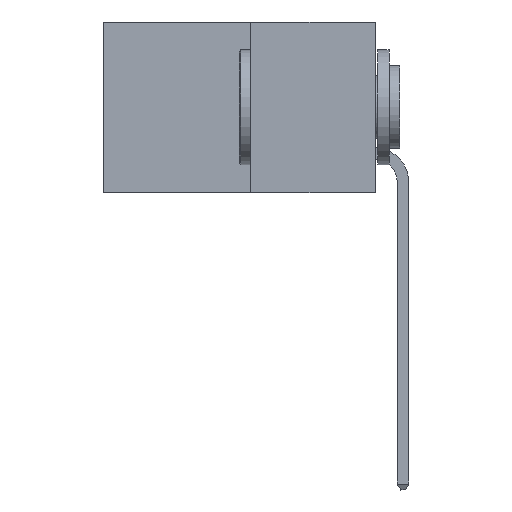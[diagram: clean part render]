
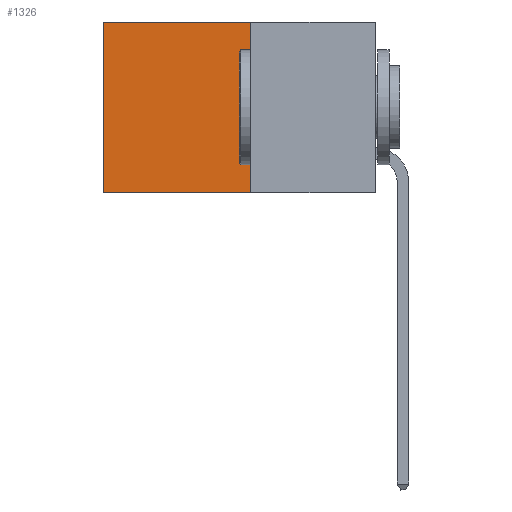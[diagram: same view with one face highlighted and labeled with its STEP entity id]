
A CAD part, left-side view. The second image highlights one B-rep face of the part: STEP entity #1326.
In plain terms, the highlighted planar face has unit normal (-1, 0, 0).
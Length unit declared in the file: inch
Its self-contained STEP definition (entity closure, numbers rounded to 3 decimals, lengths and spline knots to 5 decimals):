
#985 = AXIS2_PLACEMENT_3D ( 'NONE', #12984, #8369, #6080 ) ;
#992 = CARTESIAN_POINT ( 'NONE',  ( 0.277, 0.59, 0. ) ) ;
#1101 = VERTEX_POINT ( 'NONE', #992 ) ;
#1326 = ADVANCED_FACE ( 'NONE', ( #7805 ), #9243, .F. ) ;
#1592 = DIRECTION ( 'NONE',  ( 0., 1., 0. ) ) ;
#2831 = LINE ( 'NONE', #6170, #10589 ) ;
#2995 = VECTOR ( 'NONE', #11701, 39.37008 ) ;
#3074 = EDGE_LOOP ( 'NONE', ( #8275, #7763, #12031, #8134 ) ) ;
#3291 = CARTESIAN_POINT ( 'NONE',  ( 0.277, 0.59, -0.37 ) ) ;
#3334 = LINE ( 'NONE', #3291, #2995 ) ;
#4311 = CARTESIAN_POINT ( 'NONE',  ( 0.277, 0.59, -0.37 ) ) ;
#5219 = LINE ( 'NONE', #6321, #10451 ) ;
#6080 = DIRECTION ( 'NONE',  ( 0., 0., -1. ) ) ;
#6170 = CARTESIAN_POINT ( 'NONE',  ( 0.277, 0.27, -0.37 ) ) ;
#6261 = CARTESIAN_POINT ( 'NONE',  ( 0.277, 0.27, 0. ) ) ;
#6321 = CARTESIAN_POINT ( 'NONE',  ( 0.277, 0.27, -0.37 ) ) ;
#7609 = VECTOR ( 'NONE', #1592, 39.37008 ) ;
#7763 = ORIENTED_EDGE ( 'NONE', *, *, #11565, .F. ) ;
#7805 = FACE_OUTER_BOUND ( 'NONE', #3074, .T. ) ;
#8034 = VERTEX_POINT ( 'NONE', #4311 ) ;
#8134 = ORIENTED_EDGE ( 'NONE', *, *, #8352, .T. ) ;
#8275 = ORIENTED_EDGE ( 'NONE', *, *, #11712, .T. ) ;
#8352 = EDGE_CURVE ( 'NONE', #10520, #1101, #10449, .T. ) ;
#8369 = DIRECTION ( 'NONE',  ( 1., 0., 0. ) ) ;
#9243 = PLANE ( 'NONE',  #985 ) ;
#10057 = CARTESIAN_POINT ( 'NONE',  ( 0.277, 0.27, -0.37 ) ) ;
#10449 = LINE ( 'NONE', #11997, #7609 ) ;
#10451 = VECTOR ( 'NONE', #12676, 39.37008 ) ;
#10520 = VERTEX_POINT ( 'NONE', #6261 ) ;
#10532 = EDGE_CURVE ( 'NONE', #10520, #11343, #5219, .T. ) ;
#10589 = VECTOR ( 'NONE', #12503, 39.37008 ) ;
#11343 = VERTEX_POINT ( 'NONE', #10057 ) ;
#11565 = EDGE_CURVE ( 'NONE', #11343, #8034, #2831, .T. ) ;
#11701 = DIRECTION ( 'NONE',  ( 0., 0., -1. ) ) ;
#11712 = EDGE_CURVE ( 'NONE', #1101, #8034, #3334, .T. ) ;
#11997 = CARTESIAN_POINT ( 'NONE',  ( 0.277, 0.27, 0. ) ) ;
#12031 = ORIENTED_EDGE ( 'NONE', *, *, #10532, .F. ) ;
#12503 = DIRECTION ( 'NONE',  ( 0., 1., 0. ) ) ;
#12676 = DIRECTION ( 'NONE',  ( 0., 0., -1. ) ) ;
#12984 = CARTESIAN_POINT ( 'NONE',  ( 0.277, 0.27, -0.37 ) ) ;
